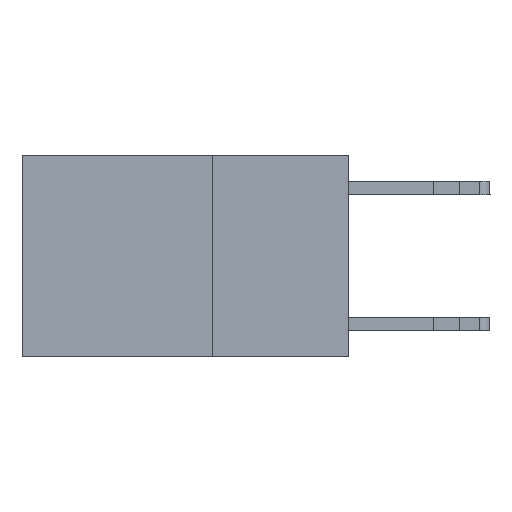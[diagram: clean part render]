
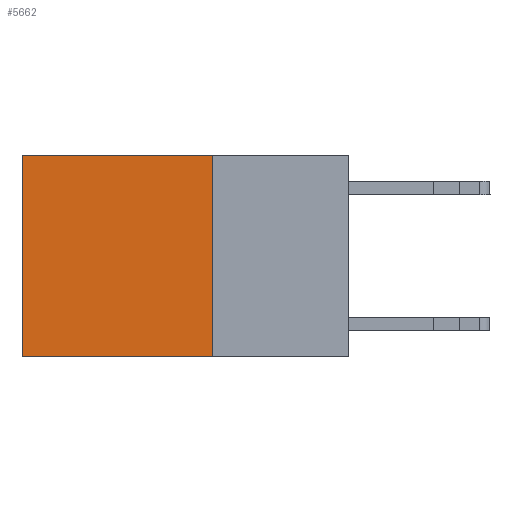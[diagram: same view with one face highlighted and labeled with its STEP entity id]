
A CAD part, left-side view. The second image highlights one B-rep face of the part: STEP entity #5662.
In plain terms, the highlighted planar face has unit normal (-1, 0, 0).
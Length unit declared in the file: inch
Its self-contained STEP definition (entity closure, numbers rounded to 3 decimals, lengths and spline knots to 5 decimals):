
#810 = VERTEX_POINT ( 'NONE', #12060 ) ;
#1352 = EDGE_CURVE ( 'NONE', #10713, #7283, #11916, .T. ) ;
#2348 = CARTESIAN_POINT ( 'NONE',  ( 0.2625, 0.6, 0. ) ) ;
#2416 = ORIENTED_EDGE ( 'NONE', *, *, #9387, .F. ) ;
#2587 = CARTESIAN_POINT ( 'NONE',  ( 0.2625, 0.6, 0. ) ) ;
#3402 = CARTESIAN_POINT ( 'NONE',  ( 0.2625, 0.25, -0.37 ) ) ;
#4068 = CARTESIAN_POINT ( 'NONE',  ( 0.2625, 0.25, 0. ) ) ;
#4812 = CARTESIAN_POINT ( 'NONE',  ( 0.2625, 0.25, 0. ) ) ;
#4941 = ORIENTED_EDGE ( 'NONE', *, *, #10556, .T. ) ;
#4972 = LINE ( 'NONE', #2348, #13546 ) ;
#5350 = LINE ( 'NONE', #4812, #13569 ) ;
#5662 = ADVANCED_FACE ( 'NONE', ( #11899 ), #11161, .F. ) ;
#5804 = CARTESIAN_POINT ( 'NONE',  ( 0.2625, 0.25, 0. ) ) ;
#5895 = ORIENTED_EDGE ( 'NONE', *, *, #9646, .T. ) ;
#6225 = VERTEX_POINT ( 'NONE', #2587 ) ;
#6812 = EDGE_LOOP ( 'NONE', ( #4941, #2416, #8129, #5895 ) ) ;
#6901 = VECTOR ( 'NONE', #10086, 39.37008 ) ;
#6926 = DIRECTION ( 'NONE',  ( 0., 0., -1. ) ) ;
#7283 = VERTEX_POINT ( 'NONE', #8767 ) ;
#8129 = ORIENTED_EDGE ( 'NONE', *, *, #1352, .F. ) ;
#8767 = CARTESIAN_POINT ( 'NONE',  ( 0.2625, 0.25, -0.37 ) ) ;
#8836 = DIRECTION ( 'NONE',  ( 0., 0., -1. ) ) ;
#9387 = EDGE_CURVE ( 'NONE', #7283, #810, #13737, .T. ) ;
#9646 = EDGE_CURVE ( 'NONE', #10713, #6225, #5350, .T. ) ;
#10086 = DIRECTION ( 'NONE',  ( 0., 0., -1. ) ) ;
#10556 = EDGE_CURVE ( 'NONE', #6225, #810, #4972, .T. ) ;
#10713 = VERTEX_POINT ( 'NONE', #13205 ) ;
#10941 = VECTOR ( 'NONE', #12066, 39.37008 ) ;
#11113 = AXIS2_PLACEMENT_3D ( 'NONE', #5804, #13286, #6926 ) ;
#11161 = PLANE ( 'NONE',  #11113 ) ;
#11899 = FACE_OUTER_BOUND ( 'NONE', #6812, .T. ) ;
#11916 = LINE ( 'NONE', #4068, #6901 ) ;
#12060 = CARTESIAN_POINT ( 'NONE',  ( 0.2625, 0.6, -0.37 ) ) ;
#12066 = DIRECTION ( 'NONE',  ( 0., 1., 0. ) ) ;
#13205 = CARTESIAN_POINT ( 'NONE',  ( 0.2625, 0.25, 0. ) ) ;
#13286 = DIRECTION ( 'NONE',  ( 1., 0., 0. ) ) ;
#13427 = DIRECTION ( 'NONE',  ( 0., 1., 0. ) ) ;
#13546 = VECTOR ( 'NONE', #8836, 39.37008 ) ;
#13569 = VECTOR ( 'NONE', #13427, 39.37008 ) ;
#13737 = LINE ( 'NONE', #3402, #10941 ) ;
